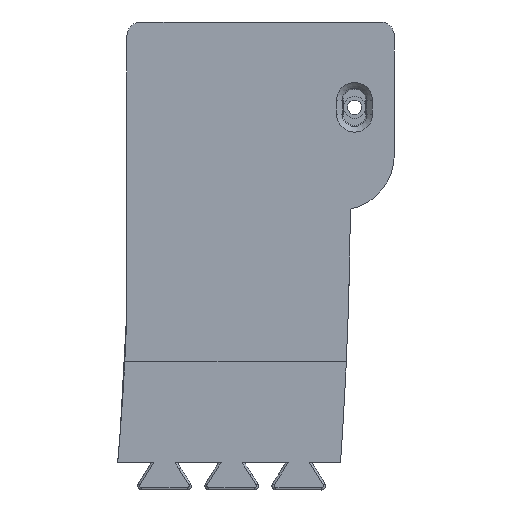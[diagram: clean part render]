
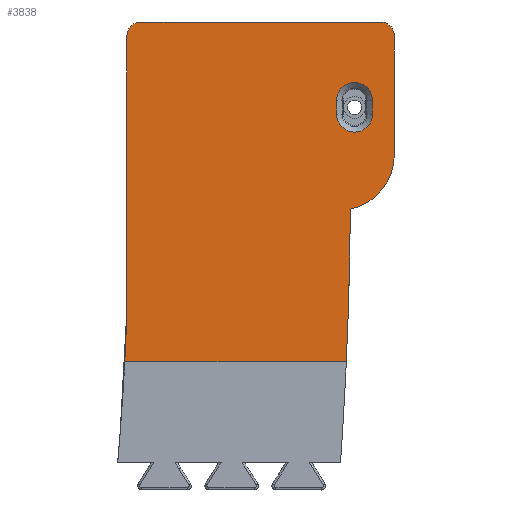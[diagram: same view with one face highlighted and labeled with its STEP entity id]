
A CAD part, front view. The second image highlights one B-rep face of the part: STEP entity #3838.
In plain terms, the highlighted planar face has unit normal (0, -1, 0).
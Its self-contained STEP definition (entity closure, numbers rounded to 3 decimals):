
#23=FACE_BOUND('',#649,.T.);
#221=CIRCLE('',#4112,949.);
#238=CIRCLE('',#4141,1465.281);
#239=CIRCLE('',#4157,5.);
#240=CIRCLE('',#4158,20.);
#241=CIRCLE('',#4159,5.);
#242=CIRCLE('',#4160,6.439);
#243=CIRCLE('',#4161,6.439);
#422=FACE_OUTER_BOUND('',#648,.T.);
#648=EDGE_LOOP('',(#3011,#3012,#3013,#3014,#3015,#3016,#3017,#3018,#3019,
#3020));
#649=EDGE_LOOP('',(#3021,#3022,#3023,#3024));
#905=LINE('',#5676,#1235);
#1000=LINE('',#7055,#1330);
#1001=LINE('',#7058,#1331);
#1002=LINE('',#7062,#1332);
#1003=LINE('',#7065,#1333);
#1004=LINE('',#7068,#1334);
#1005=LINE('',#7072,#1335);
#1235=VECTOR('',#4433,10.);
#1330=VECTOR('',#4854,10.);
#1331=VECTOR('',#4857,10.);
#1332=VECTOR('',#4860,10.);
#1333=VECTOR('',#4863,10.);
#1334=VECTOR('',#4864,10.);
#1335=VECTOR('',#4867,10.);
#1592=VERTEX_POINT('',#5673);
#1593=VERTEX_POINT('',#5675);
#1673=VERTEX_POINT('',#6659);
#1704=VERTEX_POINT('',#7023);
#1705=VERTEX_POINT('',#7053);
#1706=VERTEX_POINT('',#7054);
#1707=VERTEX_POINT('',#7056);
#1708=VERTEX_POINT('',#7059);
#1709=VERTEX_POINT('',#7061);
#1710=VERTEX_POINT('',#7063);
#1711=VERTEX_POINT('',#7066);
#1712=VERTEX_POINT('',#7067);
#1713=VERTEX_POINT('',#7069);
#1714=VERTEX_POINT('',#7071);
#1956=EDGE_CURVE('',#1593,#1592,#905,.T.);
#2110=EDGE_CURVE('',#1673,#1593,#221,.T.);
#2158=EDGE_CURVE('',#1592,#1704,#238,.T.);
#2171=EDGE_CURVE('',#1705,#1706,#1000,.T.);
#2172=EDGE_CURVE('',#1707,#1705,#239,.T.);
#2173=EDGE_CURVE('',#1707,#1673,#1001,.T.);
#2174=EDGE_CURVE('',#1708,#1704,#240,.T.);
#2175=EDGE_CURVE('',#1709,#1708,#1002,.T.);
#2176=EDGE_CURVE('',#1710,#1709,#241,.T.);
#2177=EDGE_CURVE('',#1706,#1710,#1003,.T.);
#2178=EDGE_CURVE('',#1711,#1712,#1004,.T.);
#2179=EDGE_CURVE('',#1712,#1713,#242,.T.);
#2180=EDGE_CURVE('',#1713,#1714,#1005,.T.);
#2181=EDGE_CURVE('',#1714,#1711,#243,.T.);
#3011=ORIENTED_EDGE('',*,*,#2171,.F.);
#3012=ORIENTED_EDGE('',*,*,#2172,.F.);
#3013=ORIENTED_EDGE('',*,*,#2173,.T.);
#3014=ORIENTED_EDGE('',*,*,#2110,.T.);
#3015=ORIENTED_EDGE('',*,*,#1956,.T.);
#3016=ORIENTED_EDGE('',*,*,#2158,.T.);
#3017=ORIENTED_EDGE('',*,*,#2174,.F.);
#3018=ORIENTED_EDGE('',*,*,#2175,.F.);
#3019=ORIENTED_EDGE('',*,*,#2176,.F.);
#3020=ORIENTED_EDGE('',*,*,#2177,.F.);
#3021=ORIENTED_EDGE('',*,*,#2178,.T.);
#3022=ORIENTED_EDGE('',*,*,#2179,.T.);
#3023=ORIENTED_EDGE('',*,*,#2180,.T.);
#3024=ORIENTED_EDGE('',*,*,#2181,.T.);
#3672=PLANE('',#4156);
#3838=ADVANCED_FACE('',(#422,#23),#3672,.T.);
#4112=AXIS2_PLACEMENT_3D('',#6660,#4740,#4741);
#4141=AXIS2_PLACEMENT_3D('',#7025,#4810,#4811);
#4156=AXIS2_PLACEMENT_3D('',#7052,#4852,#4853);
#4157=AXIS2_PLACEMENT_3D('',#7057,#4855,#4856);
#4158=AXIS2_PLACEMENT_3D('',#7060,#4858,#4859);
#4159=AXIS2_PLACEMENT_3D('',#7064,#4861,#4862);
#4160=AXIS2_PLACEMENT_3D('',#7070,#4865,#4866);
#4161=AXIS2_PLACEMENT_3D('',#7073,#4868,#4869);
#4433=DIRECTION('',(1.,0.,0.));
#4740=DIRECTION('center_axis',(0.,1.,0.));
#4741=DIRECTION('ref_axis',(1.,0.,-0.031));
#4810=DIRECTION('center_axis',(0.,-1.,0.));
#4811=DIRECTION('ref_axis',(1.,0.,-0.008));
#4852=DIRECTION('center_axis',(0.,-1.,0.));
#4853=DIRECTION('ref_axis',(1.,0.,0.));
#4854=DIRECTION('',(1.,0.,0.));
#4855=DIRECTION('center_axis',(0.,1.,0.));
#4856=DIRECTION('ref_axis',(-0.707,0.,0.707));
#4857=DIRECTION('',(0.,0.,-1.));
#4858=DIRECTION('center_axis',(0.,1.,0.));
#4859=DIRECTION('ref_axis',(0.208,0.,-0.978));
#4860=DIRECTION('',(0.,0.,-1.));
#4861=DIRECTION('center_axis',(0.,1.,0.));
#4862=DIRECTION('ref_axis',(0.707,0.,0.707));
#4863=DIRECTION('',(1.,0.,0.));
#4864=DIRECTION('',(0.,0.,1.));
#4865=DIRECTION('center_axis',(0.,1.,0.));
#4866=DIRECTION('ref_axis',(1.,0.,0.));
#4867=DIRECTION('',(0.,0.,-1.));
#4868=DIRECTION('center_axis',(0.,1.,0.));
#4869=DIRECTION('ref_axis',(-1.,0.,0.));
#5673=CARTESIAN_POINT('',(-21.454,6.118,-44.965));
#5675=CARTESIAN_POINT('',(-101.234,6.118,-44.965));
#5676=CARTESIAN_POINT('',(-106.432,6.118,-44.965));
#6659=CARTESIAN_POINT('',(-100.44,6.118,-25.509));
#6660=CARTESIAN_POINT('Origin',(-1048.998,6.118,3.472));
#7023=CARTESIAN_POINT('',(-20.,6.118,10.));
#7025=CARTESIAN_POINT('Origin',(-1485.238,6.118,21.265));
#7052=CARTESIAN_POINT('Origin',(-73.595,6.118,-92.256));
#7053=CARTESIAN_POINT('',(-95.44,6.118,77.408));
#7054=CARTESIAN_POINT('',(-91.44,6.118,77.408));
#7055=CARTESIAN_POINT('',(-91.44,6.118,77.408));
#7056=CARTESIAN_POINT('',(-100.44,6.118,72.408));
#7057=CARTESIAN_POINT('Origin',(-95.44,6.118,72.408));
#7058=CARTESIAN_POINT('',(-100.44,6.118,14.491));
#7059=CARTESIAN_POINT('',(-4.16,6.118,29.563));
#7060=CARTESIAN_POINT('Origin',(-24.16,6.118,29.563));
#7061=CARTESIAN_POINT('',(-4.16,6.118,72.408));
#7062=CARTESIAN_POINT('',(-4.16,6.118,-37.278));
#7063=CARTESIAN_POINT('',(-9.16,6.118,77.408));
#7064=CARTESIAN_POINT('Origin',(-9.16,6.118,72.408));
#7065=CARTESIAN_POINT('',(-9.16,6.118,77.408));
#7066=CARTESIAN_POINT('',(-24.93,6.118,44.172));
#7067=CARTESIAN_POINT('',(-24.93,6.118,49.176));
#7068=CARTESIAN_POINT('',(-24.93,6.118,65.879));
#7069=CARTESIAN_POINT('',(-12.053,6.118,49.176));
#7070=CARTESIAN_POINT('Origin',(-18.491,6.118,49.176));
#7071=CARTESIAN_POINT('',(-12.053,6.118,44.172));
#7072=CARTESIAN_POINT('',(-12.053,6.118,68.38));
#7073=CARTESIAN_POINT('Origin',(-18.491,6.118,44.172));
